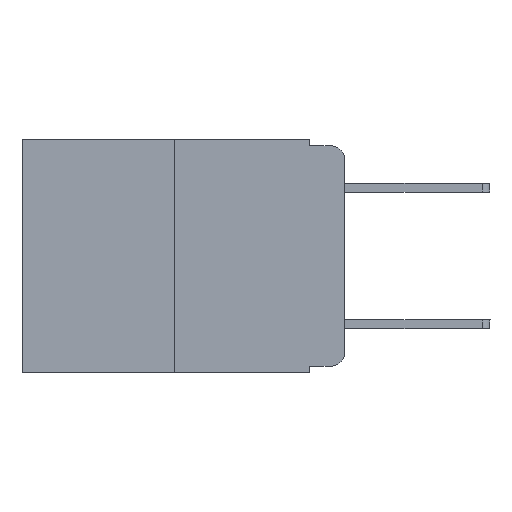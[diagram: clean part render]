
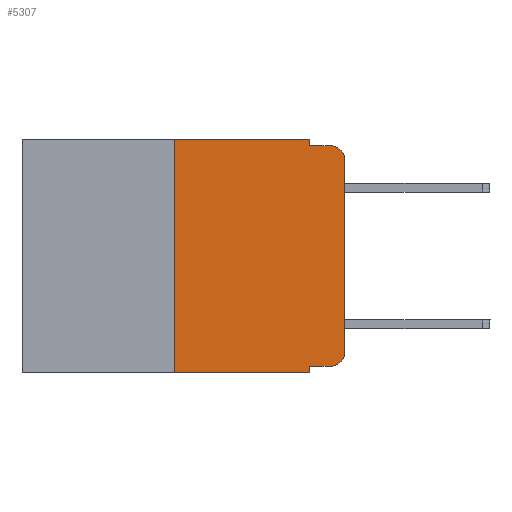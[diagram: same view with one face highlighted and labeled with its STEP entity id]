
A CAD part, left-side view. The second image highlights one B-rep face of the part: STEP entity #5307.
In plain terms, the highlighted planar face has unit normal (-1, 0, 0).
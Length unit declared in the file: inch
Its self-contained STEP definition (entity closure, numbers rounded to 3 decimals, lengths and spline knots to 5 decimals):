
#407 = VECTOR ( 'NONE', #5111, 39.37008 ) ;
#514 = EDGE_CURVE ( 'NONE', #16711, #4313, #1455, .T. ) ;
#739 = CARTESIAN_POINT ( 'NONE',  ( 0., 0.02, -0.01 ) ) ;
#829 = VECTOR ( 'NONE', #22387, 39.37008 ) ;
#844 = VERTEX_POINT ( 'NONE', #16832 ) ;
#1177 = DIRECTION ( 'NONE',  ( 1., 0., 0. ) ) ;
#1302 = VERTEX_POINT ( 'NONE', #14114 ) ;
#1455 = LINE ( 'NONE', #9369, #3250 ) ;
#1630 = DIRECTION ( 'NONE',  ( 0., 0., 1. ) ) ;
#1740 = CIRCLE ( 'NONE', #5121, 0.02 ) ;
#1832 = EDGE_CURVE ( 'NONE', #1302, #4600, #1740, .T. ) ;
#2132 = LINE ( 'NONE', #21981, #11655 ) ;
#2528 = ORIENTED_EDGE ( 'NONE', *, *, #18280, .T. ) ;
#2560 = ORIENTED_EDGE ( 'NONE', *, *, #514, .F. ) ;
#2636 = EDGE_CURVE ( 'NONE', #16613, #7723, #2132, .T. ) ;
#2711 = VERTEX_POINT ( 'NONE', #6357 ) ;
#2944 = DIRECTION ( 'NONE',  ( -1., 0., 0. ) ) ;
#3034 = LINE ( 'NONE', #6790, #10505 ) ;
#3250 = VECTOR ( 'NONE', #1630, 39.37008 ) ;
#3311 = EDGE_CURVE ( 'NONE', #4313, #11320, #21246, .T. ) ;
#3711 = LINE ( 'NONE', #6989, #407 ) ;
#4270 = AXIS2_PLACEMENT_3D ( 'NONE', #21911, #2944, #12626 ) ;
#4285 = ORIENTED_EDGE ( 'NONE', *, *, #9976, .F. ) ;
#4313 = VERTEX_POINT ( 'NONE', #7355 ) ;
#4600 = VERTEX_POINT ( 'NONE', #7213 ) ;
#4851 = CARTESIAN_POINT ( 'NONE',  ( 0., 0.051, -0.333 ) ) ;
#5104 = CARTESIAN_POINT ( 'NONE',  ( 0., 0.473, 0. ) ) ;
#5111 = DIRECTION ( 'NONE',  ( 0., -1., 0. ) ) ;
#5121 = AXIS2_PLACEMENT_3D ( 'NONE', #17959, #14303, #20154 ) ;
#5307 = ADVANCED_FACE ( 'NONE', ( #16928 ), #12607, .F. ) ;
#5308 = DIRECTION ( 'NONE',  ( 0., 0., -1. ) ) ;
#5313 = EDGE_CURVE ( 'NONE', #17909, #1302, #14851, .T. ) ;
#5887 = EDGE_CURVE ( 'NONE', #4600, #844, #24370, .T. ) ;
#6357 = CARTESIAN_POINT ( 'NONE',  ( 0., 0.051, -0.343 ) ) ;
#6790 = CARTESIAN_POINT ( 'NONE',  ( 0., 0.051, 0. ) ) ;
#6989 = CARTESIAN_POINT ( 'NONE',  ( 0., 0.473, -0.343 ) ) ;
#7213 = CARTESIAN_POINT ( 'NONE',  ( 0., 0., -0.313 ) ) ;
#7355 = CARTESIAN_POINT ( 'NONE',  ( 0., 0.25, 0. ) ) ;
#7414 = CARTESIAN_POINT ( 'NONE',  ( 0., 0.25, -0.343 ) ) ;
#7723 = VERTEX_POINT ( 'NONE', #739 ) ;
#7902 = EDGE_CURVE ( 'NONE', #11320, #16613, #3034, .T. ) ;
#8386 = CIRCLE ( 'NONE', #4270, 0.02 ) ;
#8814 = ORIENTED_EDGE ( 'NONE', *, *, #5887, .T. ) ;
#9369 = CARTESIAN_POINT ( 'NONE',  ( 0., 0.25, 0. ) ) ;
#9414 = CARTESIAN_POINT ( 'NONE',  ( 0., 0.051, -0.01 ) ) ;
#9543 = ORIENTED_EDGE ( 'NONE', *, *, #3311, .F. ) ;
#9584 = CARTESIAN_POINT ( 'NONE',  ( 0., 0.473, 0. ) ) ;
#9622 = EDGE_CURVE ( 'NONE', #844, #7723, #8386, .T. ) ;
#9976 = EDGE_CURVE ( 'NONE', #17909, #2711, #17044, .T. ) ;
#10201 = DIRECTION ( 'NONE',  ( 0., -1., 0. ) ) ;
#10505 = VECTOR ( 'NONE', #5308, 39.37008 ) ;
#11000 = CARTESIAN_POINT ( 'NONE',  ( 0., 0., 0. ) ) ;
#11320 = VERTEX_POINT ( 'NONE', #13079 ) ;
#11542 = AXIS2_PLACEMENT_3D ( 'NONE', #5104, #1177, #14428 ) ;
#11655 = VECTOR ( 'NONE', #10201, 39.37008 ) ;
#12607 = PLANE ( 'NONE',  #11542 ) ;
#12626 = DIRECTION ( 'NONE',  ( 0., 0., -1. ) ) ;
#12717 = ORIENTED_EDGE ( 'NONE', *, *, #9622, .T. ) ;
#13079 = CARTESIAN_POINT ( 'NONE',  ( 0., 0.051, 0. ) ) ;
#14114 = CARTESIAN_POINT ( 'NONE',  ( 0., 0.02, -0.333 ) ) ;
#14303 = DIRECTION ( 'NONE',  ( -1., 0., 0. ) ) ;
#14428 = DIRECTION ( 'NONE',  ( 0., 0., -1. ) ) ;
#14851 = LINE ( 'NONE', #4851, #829 ) ;
#14981 = DIRECTION ( 'NONE',  ( 0., 0., -1. ) ) ;
#15153 = EDGE_LOOP ( 'NONE', ( #8814, #12717, #15621, #20677, #9543, #2560, #2528, #4285, #20609, #18847 ) ) ;
#15271 = DIRECTION ( 'NONE',  ( 0., -1., 0. ) ) ;
#15621 = ORIENTED_EDGE ( 'NONE', *, *, #2636, .F. ) ;
#16613 = VERTEX_POINT ( 'NONE', #9414 ) ;
#16711 = VERTEX_POINT ( 'NONE', #7414 ) ;
#16745 = VECTOR ( 'NONE', #14981, 39.37008 ) ;
#16832 = CARTESIAN_POINT ( 'NONE',  ( 0., 0., -0.03 ) ) ;
#16886 = CARTESIAN_POINT ( 'NONE',  ( 0., 0.051, 0. ) ) ;
#16928 = FACE_OUTER_BOUND ( 'NONE', #15153, .T. ) ;
#17044 = LINE ( 'NONE', #16886, #16745 ) ;
#17051 = VECTOR ( 'NONE', #15271, 39.37008 ) ;
#17909 = VERTEX_POINT ( 'NONE', #22738 ) ;
#17959 = CARTESIAN_POINT ( 'NONE',  ( 0., 0.02, -0.313 ) ) ;
#18280 = EDGE_CURVE ( 'NONE', #16711, #2711, #3711, .T. ) ;
#18847 = ORIENTED_EDGE ( 'NONE', *, *, #1832, .T. ) ;
#20154 = DIRECTION ( 'NONE',  ( 0., 0., -1. ) ) ;
#20535 = DIRECTION ( 'NONE',  ( 0., 0., 1. ) ) ;
#20609 = ORIENTED_EDGE ( 'NONE', *, *, #5313, .T. ) ;
#20677 = ORIENTED_EDGE ( 'NONE', *, *, #7902, .F. ) ;
#21246 = LINE ( 'NONE', #9584, #17051 ) ;
#21911 = CARTESIAN_POINT ( 'NONE',  ( 0., 0.02, -0.03 ) ) ;
#21981 = CARTESIAN_POINT ( 'NONE',  ( 0., 0.051, -0.01 ) ) ;
#22292 = VECTOR ( 'NONE', #20535, 39.37008 ) ;
#22387 = DIRECTION ( 'NONE',  ( 0., -1., 0. ) ) ;
#22738 = CARTESIAN_POINT ( 'NONE',  ( 0., 0.051, -0.333 ) ) ;
#24370 = LINE ( 'NONE', #11000, #22292 ) ;
